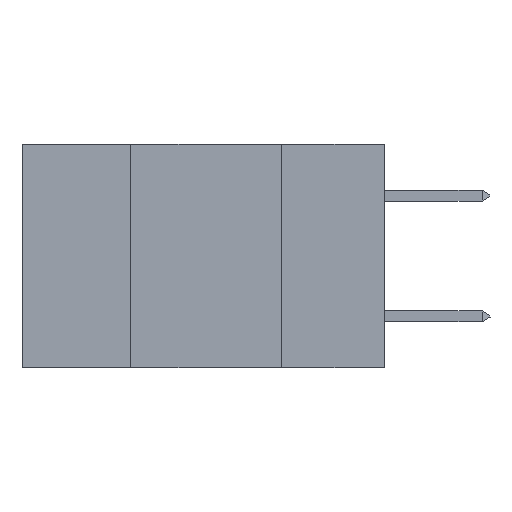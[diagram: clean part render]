
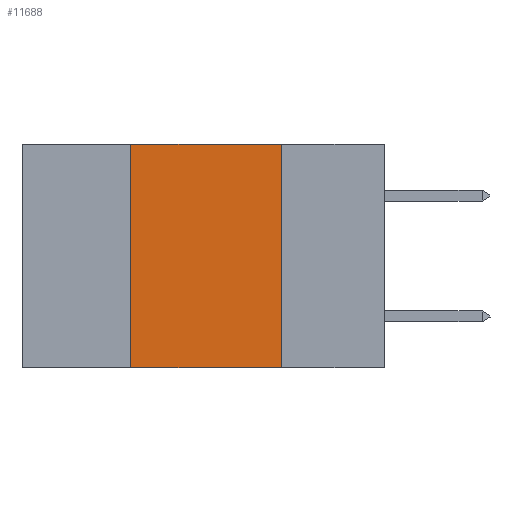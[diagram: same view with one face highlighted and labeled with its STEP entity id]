
A CAD part, left-side view. The second image highlights one B-rep face of the part: STEP entity #11688.
In plain terms, the highlighted planar face has unit normal (-1, 0, 0).
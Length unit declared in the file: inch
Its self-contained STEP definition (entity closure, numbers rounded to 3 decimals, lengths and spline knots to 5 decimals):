
#768 = ORIENTED_EDGE ( 'NONE', *, *, #16074, .F. ) ;
#882 = LINE ( 'NONE', #6553, #23520 ) ;
#1042 = VERTEX_POINT ( 'NONE', #8827 ) ;
#1763 = CARTESIAN_POINT ( 'NONE',  ( 0., 0.17, -0.37 ) ) ;
#3209 = PLANE ( 'NONE',  #11299 ) ;
#3319 = LINE ( 'NONE', #19830, #24529 ) ;
#3458 = CARTESIAN_POINT ( 'NONE',  ( 0., 0.6, -0.37 ) ) ;
#4526 = FACE_OUTER_BOUND ( 'NONE', #25658, .T. ) ;
#6487 = LINE ( 'NONE', #3458, #24727 ) ;
#6553 = CARTESIAN_POINT ( 'NONE',  ( 0., 0.17, 0. ) ) ;
#6600 = LINE ( 'NONE', #8585, #20405 ) ;
#6661 = DIRECTION ( 'NONE',  ( 0., 0., 1. ) ) ;
#7886 = DIRECTION ( 'NONE',  ( 0., -1., 0. ) ) ;
#8011 = VERTEX_POINT ( 'NONE', #8543 ) ;
#8543 = CARTESIAN_POINT ( 'NONE',  ( 0., 0.17, 0. ) ) ;
#8585 = CARTESIAN_POINT ( 'NONE',  ( 0., 0.6, 0. ) ) ;
#8827 = CARTESIAN_POINT ( 'NONE',  ( 0., 0.42, 0. ) ) ;
#10685 = EDGE_CURVE ( 'NONE', #8011, #23946, #882, .T. ) ;
#11299 = AXIS2_PLACEMENT_3D ( 'NONE', #13929, #24924, #20248 ) ;
#11688 = ADVANCED_FACE ( 'NONE', ( #4526 ), #3209, .F. ) ;
#13929 = CARTESIAN_POINT ( 'NONE',  ( 0., 0.6, 0. ) ) ;
#14551 = VERTEX_POINT ( 'NONE', #27193 ) ;
#15105 = ORIENTED_EDGE ( 'NONE', *, *, #22595, .T. ) ;
#16000 = ORIENTED_EDGE ( 'NONE', *, *, #25488, .F. ) ;
#16074 = EDGE_CURVE ( 'NONE', #1042, #8011, #6600, .T. ) ;
#19830 = CARTESIAN_POINT ( 'NONE',  ( 0., 0.42, 0. ) ) ;
#20248 = DIRECTION ( 'NONE',  ( 0., 0., -1. ) ) ;
#20405 = VECTOR ( 'NONE', #23672, 39.37008 ) ;
#22595 = EDGE_CURVE ( 'NONE', #14551, #23946, #6487, .T. ) ;
#23520 = VECTOR ( 'NONE', #23913, 39.37008 ) ;
#23672 = DIRECTION ( 'NONE',  ( 0., -1., 0. ) ) ;
#23913 = DIRECTION ( 'NONE',  ( 0., 0., -1. ) ) ;
#23946 = VERTEX_POINT ( 'NONE', #1763 ) ;
#24529 = VECTOR ( 'NONE', #6661, 39.37008 ) ;
#24727 = VECTOR ( 'NONE', #7886, 39.37008 ) ;
#24924 = DIRECTION ( 'NONE',  ( 1., 0., 0. ) ) ;
#25258 = ORIENTED_EDGE ( 'NONE', *, *, #10685, .F. ) ;
#25488 = EDGE_CURVE ( 'NONE', #14551, #1042, #3319, .T. ) ;
#25658 = EDGE_LOOP ( 'NONE', ( #25258, #768, #16000, #15105 ) ) ;
#27193 = CARTESIAN_POINT ( 'NONE',  ( 0., 0.42, -0.37 ) ) ;
